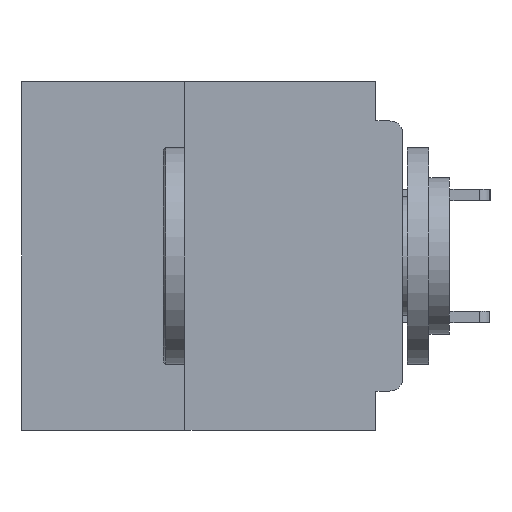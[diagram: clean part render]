
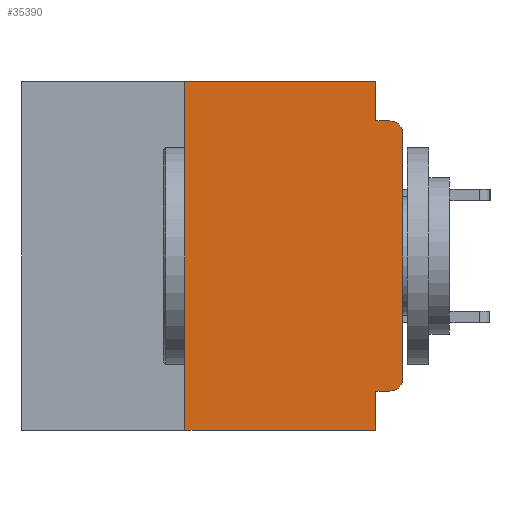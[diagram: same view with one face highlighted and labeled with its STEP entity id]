
A CAD part, left-side view. The second image highlights one B-rep face of the part: STEP entity #35390.
In plain terms, the highlighted planar face has unit normal (-1, 0, 0).
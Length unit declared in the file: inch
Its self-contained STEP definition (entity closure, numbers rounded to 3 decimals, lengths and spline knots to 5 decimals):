
#199 = CARTESIAN_POINT ( 'NONE',  ( 0., 0.015, -0.06 ) ) ;
#548 = DIRECTION ( 'NONE',  ( 0., -1., 0. ) ) ;
#863 = VERTEX_POINT ( 'NONE', #38906 ) ;
#890 = CARTESIAN_POINT ( 'NONE',  ( 0., 0.031, -0.4 ) ) ;
#1620 = CARTESIAN_POINT ( 'NONE',  ( 0., 0.25, -0.4 ) ) ;
#1927 = PLANE ( 'NONE',  #26297 ) ;
#2025 = DIRECTION ( 'NONE',  ( 0., 0., 1. ) ) ;
#2438 = VECTOR ( 'NONE', #31432, 39.37008 ) ;
#3461 = DIRECTION ( 'NONE',  ( 0., 0., -1. ) ) ;
#4418 = LINE ( 'NONE', #34216, #28163 ) ;
#4767 = LINE ( 'NONE', #28438, #12031 ) ;
#4827 = DIRECTION ( 'NONE',  ( 0., 0., 1. ) ) ;
#5058 = VERTEX_POINT ( 'NONE', #7227 ) ;
#5127 = DIRECTION ( 'NONE',  ( 1., 0., 0. ) ) ;
#6278 = VECTOR ( 'NONE', #8734, 39.37008 ) ;
#6635 = LINE ( 'NONE', #1620, #22083 ) ;
#6757 = CARTESIAN_POINT ( 'NONE',  ( 0., 0., -0.34 ) ) ;
#6895 = AXIS2_PLACEMENT_3D ( 'NONE', #199, #22001, #3461 ) ;
#7083 = CARTESIAN_POINT ( 'NONE',  ( 0., 0.031, -0.355 ) ) ;
#7227 = CARTESIAN_POINT ( 'NONE',  ( 0., 0.031, 0. ) ) ;
#7929 = VERTEX_POINT ( 'NONE', #33325 ) ;
#8734 = DIRECTION ( 'NONE',  ( 0., 1., 0. ) ) ;
#9511 = DIRECTION ( 'NONE',  ( 0., -1., 0. ) ) ;
#10435 = EDGE_CURVE ( 'NONE', #19539, #21729, #16570, .T. ) ;
#12031 = VECTOR ( 'NONE', #548, 39.37008 ) ;
#12507 = VECTOR ( 'NONE', #2025, 39.37008 ) ;
#13350 = EDGE_CURVE ( 'NONE', #35927, #38670, #22060, .T. ) ;
#13479 = ORIENTED_EDGE ( 'NONE', *, *, #17209, .F. ) ;
#15077 = FACE_OUTER_BOUND ( 'NONE', #26762, .T. ) ;
#15608 = CARTESIAN_POINT ( 'NONE',  ( 0., 0.437, -0.4 ) ) ;
#15807 = CARTESIAN_POINT ( 'NONE',  ( 0., 0.015, -0.34 ) ) ;
#16194 = EDGE_CURVE ( 'NONE', #21729, #35927, #20742, .T. ) ;
#16202 = CARTESIAN_POINT ( 'NONE',  ( 0., 0.015, -0.355 ) ) ;
#16570 = CIRCLE ( 'NONE', #31331, 0.015 ) ;
#17209 = EDGE_CURVE ( 'NONE', #20959, #33222, #6635, .T. ) ;
#18127 = ORIENTED_EDGE ( 'NONE', *, *, #20018, .F. ) ;
#18492 = VECTOR ( 'NONE', #9511, 39.37008 ) ;
#18885 = DIRECTION ( 'NONE',  ( 0., 0., -1. ) ) ;
#19539 = VERTEX_POINT ( 'NONE', #16202 ) ;
#19955 = EDGE_CURVE ( 'NONE', #5058, #863, #4418, .T. ) ;
#20018 = EDGE_CURVE ( 'NONE', #863, #38670, #27205, .T. ) ;
#20742 = LINE ( 'NONE', #32885, #12507 ) ;
#20959 = VERTEX_POINT ( 'NONE', #27373 ) ;
#21003 = CARTESIAN_POINT ( 'NONE',  ( 0., 0., -0.355 ) ) ;
#21729 = VERTEX_POINT ( 'NONE', #6757 ) ;
#22001 = DIRECTION ( 'NONE',  ( -1., 0., 0. ) ) ;
#22060 = CIRCLE ( 'NONE', #6895, 0.015 ) ;
#22083 = VECTOR ( 'NONE', #4827, 39.37008 ) ;
#22430 = ORIENTED_EDGE ( 'NONE', *, *, #35007, .T. ) ;
#22758 = ORIENTED_EDGE ( 'NONE', *, *, #13350, .T. ) ;
#23453 = EDGE_CURVE ( 'NONE', #19539, #36393, #30904, .T. ) ;
#23727 = EDGE_CURVE ( 'NONE', #33222, #5058, #4767, .T. ) ;
#23904 = ORIENTED_EDGE ( 'NONE', *, *, #23727, .F. ) ;
#26297 = AXIS2_PLACEMENT_3D ( 'NONE', #35849, #5127, #26769 ) ;
#26762 = EDGE_LOOP ( 'NONE', ( #33813, #22758, #18127, #37650, #23904, #13479, #22430, #34690, #33464, #32821 ) ) ;
#26769 = DIRECTION ( 'NONE',  ( 0., 0., -1. ) ) ;
#27205 = LINE ( 'NONE', #28385, #2438 ) ;
#27373 = CARTESIAN_POINT ( 'NONE',  ( 0., 0.25, -0.4 ) ) ;
#28163 = VECTOR ( 'NONE', #37285, 39.37008 ) ;
#28385 = CARTESIAN_POINT ( 'NONE',  ( 0., 0., -0.045 ) ) ;
#28438 = CARTESIAN_POINT ( 'NONE',  ( 0., 0.437, 0. ) ) ;
#28884 = DIRECTION ( 'NONE',  ( 0., 0., -1. ) ) ;
#29536 = CARTESIAN_POINT ( 'NONE',  ( 0., 0., -0.06 ) ) ;
#30904 = LINE ( 'NONE', #21003, #6278 ) ;
#31331 = AXIS2_PLACEMENT_3D ( 'NONE', #15807, #37230, #18885 ) ;
#31432 = DIRECTION ( 'NONE',  ( 0., -1., 0. ) ) ;
#32821 = ORIENTED_EDGE ( 'NONE', *, *, #10435, .T. ) ;
#32885 = CARTESIAN_POINT ( 'NONE',  ( 0., 0., 0. ) ) ;
#32925 = EDGE_CURVE ( 'NONE', #36393, #7929, #39371, .T. ) ;
#33222 = VERTEX_POINT ( 'NONE', #36456 ) ;
#33325 = CARTESIAN_POINT ( 'NONE',  ( 0., 0.031, -0.4 ) ) ;
#33464 = ORIENTED_EDGE ( 'NONE', *, *, #23453, .F. ) ;
#33813 = ORIENTED_EDGE ( 'NONE', *, *, #16194, .T. ) ;
#34216 = CARTESIAN_POINT ( 'NONE',  ( 0., 0.031, 0. ) ) ;
#34690 = ORIENTED_EDGE ( 'NONE', *, *, #32925, .F. ) ;
#35007 = EDGE_CURVE ( 'NONE', #20959, #7929, #35768, .T. ) ;
#35390 = ADVANCED_FACE ( 'NONE', ( #15077 ), #1927, .F. ) ;
#35768 = LINE ( 'NONE', #15608, #18492 ) ;
#35849 = CARTESIAN_POINT ( 'NONE',  ( 0., 0.437, 0. ) ) ;
#35927 = VERTEX_POINT ( 'NONE', #29536 ) ;
#36393 = VERTEX_POINT ( 'NONE', #7083 ) ;
#36456 = CARTESIAN_POINT ( 'NONE',  ( 0., 0.25, 0. ) ) ;
#37230 = DIRECTION ( 'NONE',  ( -1., 0., 0. ) ) ;
#37285 = DIRECTION ( 'NONE',  ( 0., 0., -1. ) ) ;
#37650 = ORIENTED_EDGE ( 'NONE', *, *, #19955, .F. ) ;
#38419 = VECTOR ( 'NONE', #28884, 39.37008 ) ;
#38670 = VERTEX_POINT ( 'NONE', #39730 ) ;
#38906 = CARTESIAN_POINT ( 'NONE',  ( 0., 0.031, -0.045 ) ) ;
#39371 = LINE ( 'NONE', #890, #38419 ) ;
#39730 = CARTESIAN_POINT ( 'NONE',  ( 0., 0.015, -0.045 ) ) ;
